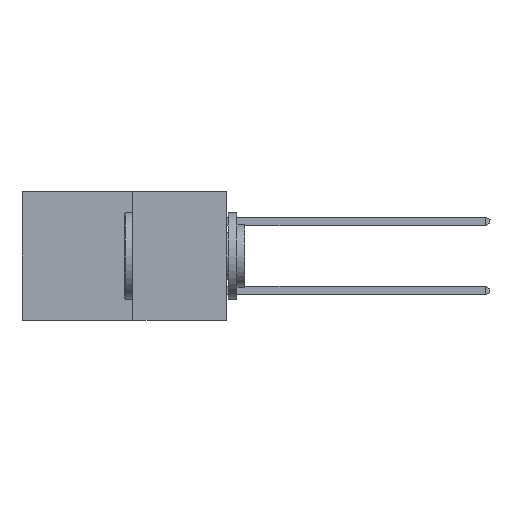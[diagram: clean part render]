
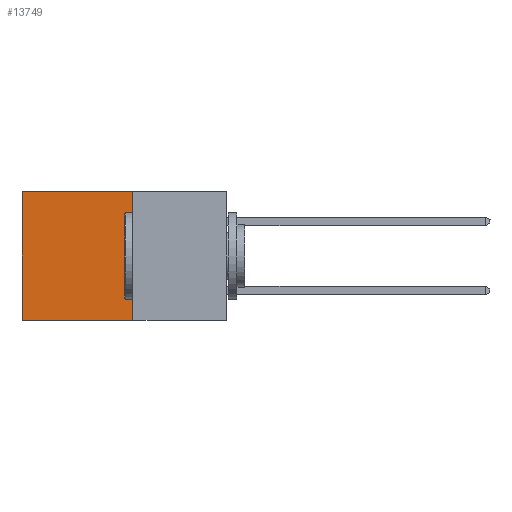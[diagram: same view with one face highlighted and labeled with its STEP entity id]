
A CAD part, left-side view. The second image highlights one B-rep face of the part: STEP entity #13749.
In plain terms, the highlighted planar face has unit normal (-1, 0, 0).
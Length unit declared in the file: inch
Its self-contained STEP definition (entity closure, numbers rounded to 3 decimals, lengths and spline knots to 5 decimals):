
#721 = VERTEX_POINT ( 'NONE', #6088 ) ;
#2352 = VECTOR ( 'NONE', #18846, 39.37008 ) ;
#2389 = VECTOR ( 'NONE', #13875, 39.37008 ) ;
#2395 = VERTEX_POINT ( 'NONE', #4900 ) ;
#3706 = CARTESIAN_POINT ( 'NONE',  ( 0.277, 0.27, -0.37 ) ) ;
#3825 = EDGE_CURVE ( 'NONE', #721, #6932, #15064, .T. ) ;
#4054 = CARTESIAN_POINT ( 'NONE',  ( 0.277, 0.27, -0.37 ) ) ;
#4900 = CARTESIAN_POINT ( 'NONE',  ( 0.277, 0.59, 0. ) ) ;
#5575 = CARTESIAN_POINT ( 'NONE',  ( 0.277, 0.27, -0.37 ) ) ;
#6088 = CARTESIAN_POINT ( 'NONE',  ( 0.277, 0.27, 0. ) ) ;
#6121 = CARTESIAN_POINT ( 'NONE',  ( 0.277, 0.59, -0.37 ) ) ;
#6304 = CARTESIAN_POINT ( 'NONE',  ( 0.277, 0.27, 0. ) ) ;
#6932 = VERTEX_POINT ( 'NONE', #5575 ) ;
#7786 = CARTESIAN_POINT ( 'NONE',  ( 0.277, 0.27, -0.37 ) ) ;
#7854 = DIRECTION ( 'NONE',  ( 1., 0., 0. ) ) ;
#8116 = ORIENTED_EDGE ( 'NONE', *, *, #12345, .T. ) ;
#8158 = ORIENTED_EDGE ( 'NONE', *, *, #18025, .F. ) ;
#8220 = ORIENTED_EDGE ( 'NONE', *, *, #3825, .F. ) ;
#8258 = EDGE_LOOP ( 'NONE', ( #8116, #8158, #8220, #8431 ) ) ;
#8431 = ORIENTED_EDGE ( 'NONE', *, *, #13093, .T. ) ;
#9369 = PLANE ( 'NONE',  #18564 ) ;
#10004 = VERTEX_POINT ( 'NONE', #12511 ) ;
#10620 = LINE ( 'NONE', #4054, #18075 ) ;
#10772 = FACE_OUTER_BOUND ( 'NONE', #8258, .T. ) ;
#11041 = DIRECTION ( 'NONE',  ( 0., 1., 0. ) ) ;
#12345 = EDGE_CURVE ( 'NONE', #2395, #10004, #18590, .T. ) ;
#12511 = CARTESIAN_POINT ( 'NONE',  ( 0.277, 0.59, -0.37 ) ) ;
#13093 = EDGE_CURVE ( 'NONE', #721, #2395, #18016, .T. ) ;
#13312 = DIRECTION ( 'NONE',  ( 0., 1., 0. ) ) ;
#13749 = ADVANCED_FACE ( 'NONE', ( #10772 ), #9369, .F. ) ;
#13875 = DIRECTION ( 'NONE',  ( 0., 0., -1. ) ) ;
#15064 = LINE ( 'NONE', #3706, #2352 ) ;
#17550 = VECTOR ( 'NONE', #11041, 39.37008 ) ;
#18016 = LINE ( 'NONE', #6304, #17550 ) ;
#18025 = EDGE_CURVE ( 'NONE', #6932, #10004, #10620, .T. ) ;
#18075 = VECTOR ( 'NONE', #13312, 39.37008 ) ;
#18445 = DIRECTION ( 'NONE',  ( 0., 0., -1. ) ) ;
#18564 = AXIS2_PLACEMENT_3D ( 'NONE', #7786, #7854, #18445 ) ;
#18590 = LINE ( 'NONE', #6121, #2389 ) ;
#18846 = DIRECTION ( 'NONE',  ( 0., 0., -1. ) ) ;
